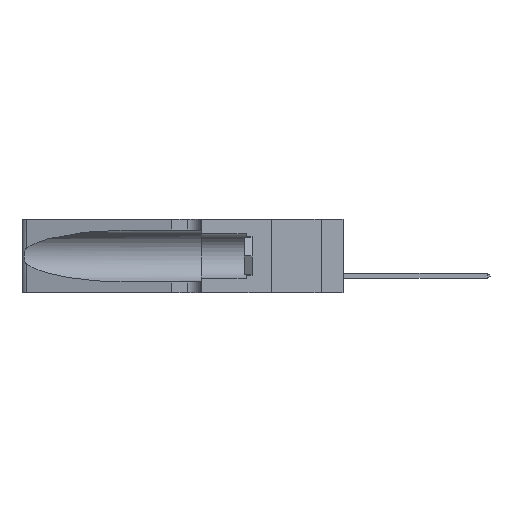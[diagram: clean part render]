
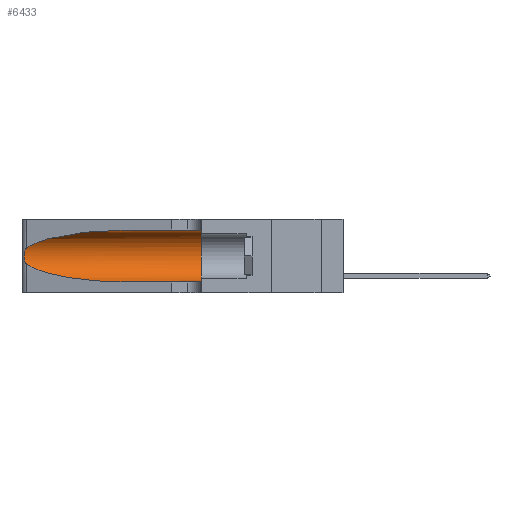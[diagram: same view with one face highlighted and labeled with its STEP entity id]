
A CAD part, left-side view. The second image highlights one B-rep face of the part: STEP entity #6433.
In plain terms, the highlighted cylindrical face has radius 3.308 mm (diameter 6.617 mm), a partial arc.
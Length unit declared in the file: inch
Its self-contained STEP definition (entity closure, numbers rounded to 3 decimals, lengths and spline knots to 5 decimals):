
#350 = DIRECTION ( 'NONE',  ( 0., -1., 0. ) ) ;
#1248 = LINE ( 'NONE', #7416, #42457 ) ;
#2106 = FACE_OUTER_BOUND ( 'NONE', #28438, .T. ) ;
#3689 = VERTEX_POINT ( 'NONE', #20102 ) ;
#5083 = CARTESIAN_POINT ( 'NONE',  ( 0.25487, 1.22718, 0.14631 ) ) ;
#5347 = CARTESIAN_POINT ( 'NONE',  ( 0.1305, 1.61858, 0.31525 ) ) ;
#6013 = AXIS2_PLACEMENT_3D ( 'NONE', #13597, #43709, #21180 ) ;
#6377 = DIRECTION ( 'NONE',  ( 0., 0., 1. ) ) ;
#6433 = ADVANCED_FACE ( 'NONE', ( #2106 ), #36851, .F. ) ;
#7416 = CARTESIAN_POINT ( 'NONE',  ( 0.1305, 1.61858, 0.05475 ) ) ;
#7913 = ORIENTED_EDGE ( 'NONE', *, *, #45753, .T. ) ;
#7954 = ORIENTED_EDGE ( 'NONE', *, *, #16989, .T. ) ;
#8245 = CARTESIAN_POINT ( 'NONE',  ( 0.26018, 1.23835, 0.19895 ) ) ;
#8536 = ORIENTED_EDGE ( 'NONE', *, *, #43954, .T. ) ;
#8636 = CARTESIAN_POINT ( 'NONE',  ( 0.1305, 0.35, 0.31525 ) ) ;
#9069 = CARTESIAN_POINT ( 'NONE',  ( 0.1305, 0.72297, 0.05475 ) ) ;
#9655 = DIRECTION ( 'NONE',  ( 0., 1., 0. ) ) ;
#9880 = CARTESIAN_POINT ( 'NONE',  ( 0.1305, 0.35, 0.05475 ) ) ;
#10362 = EDGE_CURVE ( 'NONE', #17443, #21434, #12584, .T. ) ;
#10429 = CARTESIAN_POINT ( 'NONE',  ( 0.2373, 1.15595, 0.08982 ) ) ;
#10603 = CARTESIAN_POINT ( 'NONE',  ( 0.1305, 0.72297, 0.31525 ) ) ;
#10955 =( BOUNDED_CURVE ( )  B_SPLINE_CURVE ( 3, ( #10603, #48164, #32687, #24959 ),
 .UNSPECIFIED., .F., .F. ) 
 B_SPLINE_CURVE_WITH_KNOTS ( ( 4, 4 ),
 ( 1.5708, 2.84003 ),
 .UNSPECIFIED. ) 
 CURVE ( )  GEOMETRIC_REPRESENTATION_ITEM ( )  RATIONAL_B_SPLINE_CURVE ( ( 1., 0.87, 0.87, 1. ) ) 
 REPRESENTATION_ITEM ( '' )  );
#11427 = EDGE_CURVE ( 'NONE', #3689, #17443, #32139, .T. ) ;
#11726 = CARTESIAN_POINT ( 'NONE',  ( 0.25639, 1.23186, 0.15144 ) ) ;
#11727 = CARTESIAN_POINT ( 'NONE',  ( 0.25639, 1.23184, 0.21858 ) ) ;
#11847 = ORIENTED_EDGE ( 'NONE', *, *, #10362, .F. ) ;
#12584 = CIRCLE ( 'NONE', #47112, 0.13025 ) ;
#12859 = CARTESIAN_POINT ( 'NONE',  ( 0.25856, 1.23593, 0.16098 ) ) ;
#13597 = CARTESIAN_POINT ( 'NONE',  ( 0.1305, 1.61858, 0.185 ) ) ;
#14063 = CARTESIAN_POINT ( 'NONE',  ( 0.1305, 0.72297, 0.05475 ) ) ;
#16989 = EDGE_CURVE ( 'NONE', #3689, #35891, #10955, .T. ) ;
#17088 = CARTESIAN_POINT ( 'NONE',  ( 0.1305, 0.35, 0.185 ) ) ;
#17443 = VERTEX_POINT ( 'NONE', #8636 ) ;
#19391 = CARTESIAN_POINT ( 'NONE',  ( 0.25854, 1.2359, 0.20912 ) ) ;
#19664 =( BOUNDED_CURVE ( )  B_SPLINE_CURVE ( 3, ( #36597, #10429, #40063, #14063 ),
 .UNSPECIFIED., .F., .T. ) 
 B_SPLINE_CURVE_WITH_KNOTS ( ( 4, 4 ),
 ( 3.44316, 4.71239 ),
 .UNSPECIFIED. ) 
 CURVE ( )  GEOMETRIC_REPRESENTATION_ITEM ( )  RATIONAL_B_SPLINE_CURVE ( ( 1., 0.87, 0.87, 1. ) ) 
 REPRESENTATION_ITEM ( '' )  );
#20102 = CARTESIAN_POINT ( 'NONE',  ( 0.1305, 0.72297, 0.31525 ) ) ;
#20548 = VERTEX_POINT ( 'NONE', #5083 ) ;
#20643 = CARTESIAN_POINT ( 'NONE',  ( 0.26075, 1.23896, 0.19203 ) ) ;
#21180 = DIRECTION ( 'NONE',  ( 0., 0., -1. ) ) ;
#21434 = VERTEX_POINT ( 'NONE', #9880 ) ;
#22756 = CARTESIAN_POINT ( 'NONE',  ( 0.25487, 1.22718, 0.14631 ) ) ;
#23113 = ORIENTED_EDGE ( 'NONE', *, *, #37648, .T. ) ;
#24426 = VERTEX_POINT ( 'NONE', #9069 ) ;
#24512 = CARTESIAN_POINT ( 'NONE',  ( 0.25487, 1.22718, 0.22369 ) ) ;
#24959 = CARTESIAN_POINT ( 'NONE',  ( 0.25487, 1.22718, 0.22369 ) ) ;
#24975 = CARTESIAN_POINT ( 'NONE',  ( 0.26075, 1.23896, 0.178 ) ) ;
#25297 = ORIENTED_EDGE ( 'NONE', *, *, #11427, .F. ) ;
#28438 = EDGE_LOOP ( 'NONE', ( #7954, #8536, #23113, #7913, #11847, #25297 ) ) ;
#29987 = B_SPLINE_CURVE_WITH_KNOTS ( 'NONE', 3,
 ( #36344, #33028, #11727, #31108, #19391, #8245, #20643, #24975, #32434, #12859, #34276, #11726, #34432, #22756 ),
 .UNSPECIFIED., .F., .F.,
 ( 4, 2, 2, 2, 2, 2, 4 ),
 ( 0., 0.00027, 0.00053, 0.00107, 0.0016, 0.00187, 0.00214 ),
 .UNSPECIFIED. ) ;
#31108 = CARTESIAN_POINT ( 'NONE',  ( 0.25787, 1.23484, 0.2124 ) ) ;
#32139 = LINE ( 'NONE', #5347, #47470 ) ;
#32434 = CARTESIAN_POINT ( 'NONE',  ( 0.26017, 1.23833, 0.17102 ) ) ;
#32687 = CARTESIAN_POINT ( 'NONE',  ( 0.2373, 1.15595, 0.28018 ) ) ;
#33028 = CARTESIAN_POINT ( 'NONE',  ( 0.25555, 1.22994, 0.2215 ) ) ;
#34276 = CARTESIAN_POINT ( 'NONE',  ( 0.25789, 1.23486, 0.15765 ) ) ;
#34432 = CARTESIAN_POINT ( 'NONE',  ( 0.25555, 1.22993, 0.14849 ) ) ;
#35891 = VERTEX_POINT ( 'NONE', #24512 ) ;
#36344 = CARTESIAN_POINT ( 'NONE',  ( 0.25487, 1.22718, 0.22369 ) ) ;
#36597 = CARTESIAN_POINT ( 'NONE',  ( 0.25487, 1.22718, 0.14631 ) ) ;
#36851 = CYLINDRICAL_SURFACE ( 'NONE', #6013, 0.13025 ) ;
#37648 = EDGE_CURVE ( 'NONE', #20548, #24426, #19664, .T. ) ;
#40063 = CARTESIAN_POINT ( 'NONE',  ( 0.18966, 0.96281, 0.05475 ) ) ;
#42457 = VECTOR ( 'NONE', #350, 39.37008 ) ;
#43709 = DIRECTION ( 'NONE',  ( 0., -1., 0. ) ) ;
#43954 = EDGE_CURVE ( 'NONE', #35891, #20548, #29987, .T. ) ;
#45753 = EDGE_CURVE ( 'NONE', #24426, #21434, #1248, .T. ) ;
#46517 = DIRECTION ( 'NONE',  ( 0., -1., 0. ) ) ;
#47112 = AXIS2_PLACEMENT_3D ( 'NONE', #17088, #9655, #6377 ) ;
#47470 = VECTOR ( 'NONE', #46517, 39.37008 ) ;
#48164 = CARTESIAN_POINT ( 'NONE',  ( 0.18966, 0.96281, 0.31525 ) ) ;
